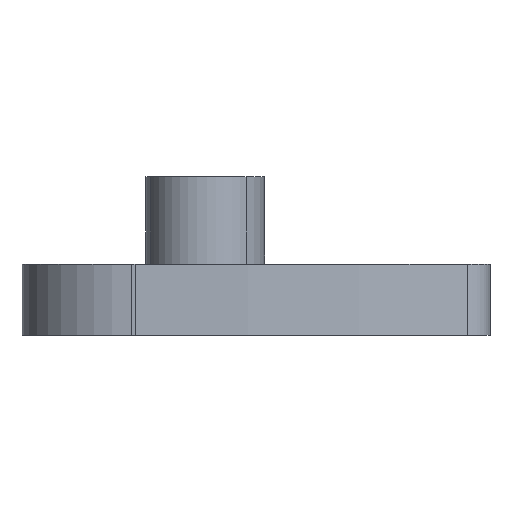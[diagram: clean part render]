
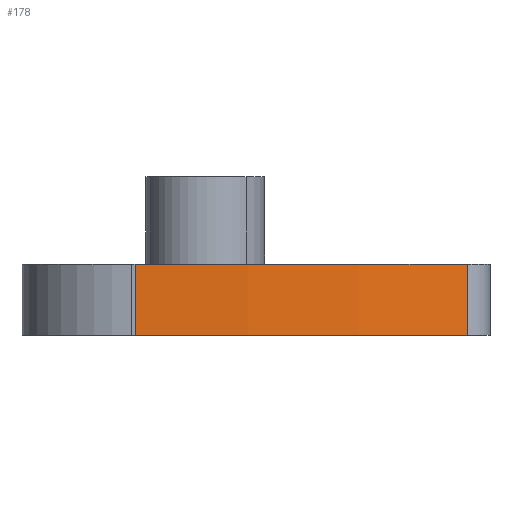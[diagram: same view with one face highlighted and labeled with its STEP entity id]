
A CAD part, left-side view. The second image highlights one B-rep face of the part: STEP entity #178.
In plain terms, the highlighted cylindrical face has radius 51.721 mm (diameter 103.442 mm), a partial arc.
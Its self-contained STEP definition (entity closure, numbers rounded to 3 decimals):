
#3 = AXIS2_PLACEMENT_3D ( 'NONE', #435, #183, #52 ) ;
#4 = CARTESIAN_POINT ( 'NONE',  ( -4.997, -12.663, 3.25 ) ) ;
#16 = DIRECTION ( 'NONE',  ( 0., 0., 1. ) ) ;
#52 = DIRECTION ( 'NONE',  ( 1., 0., 0. ) ) ;
#56 = VECTOR ( 'NONE', #476, 1000. ) ;
#168 = CIRCLE ( 'NONE', #233, 51.721 ) ;
#178 = ADVANCED_FACE ( 'NONE', ( #432 ), #405, .T. ) ;
#183 = DIRECTION ( 'NONE',  ( 0., 0., 1. ) ) ;
#191 = ORIENTED_EDGE ( 'NONE', *, *, #576, .T. ) ;
#193 = VERTEX_POINT ( 'NONE', #826 ) ;
#195 = DIRECTION ( 'NONE',  ( 0., 0., 1. ) ) ;
#225 = LINE ( 'NONE', #603, #56 ) ;
#229 = DIRECTION ( 'NONE',  ( 0., 0., 1. ) ) ;
#233 = AXIS2_PLACEMENT_3D ( 'NONE', #619, #229, #680 ) ;
#265 = LINE ( 'NONE', #471, #413 ) ;
#283 = ORIENTED_EDGE ( 'NONE', *, *, #602, .F. ) ;
#297 = CARTESIAN_POINT ( 'NONE',  ( -2.433, -27.845, 0. ) ) ;
#405 = CYLINDRICAL_SURFACE ( 'NONE', #3, 51.721 ) ;
#413 = VECTOR ( 'NONE', #16, 1000. ) ;
#432 = FACE_OUTER_BOUND ( 'NONE', #519, .T. ) ;
#435 = CARTESIAN_POINT ( 'NONE',  ( 46.715, -11.736, 0. ) ) ;
#437 = ORIENTED_EDGE ( 'NONE', *, *, #787, .F. ) ;
#464 = VERTEX_POINT ( 'NONE', #4 ) ;
#471 = CARTESIAN_POINT ( 'NONE',  ( -2.433, -27.845, 0. ) ) ;
#476 = DIRECTION ( 'NONE',  ( 0., 0., 1. ) ) ;
#519 = EDGE_LOOP ( 'NONE', ( #837, #191, #437, #283 ) ) ;
#576 = EDGE_CURVE ( 'NONE', #729, #825, #265, .T. ) ;
#584 = CARTESIAN_POINT ( 'NONE',  ( 46.715, -11.736, 3.25 ) ) ;
#588 = CARTESIAN_POINT ( 'NONE',  ( -2.433, -27.845, 3.25 ) ) ;
#602 = EDGE_CURVE ( 'NONE', #193, #464, #225, .T. ) ;
#603 = CARTESIAN_POINT ( 'NONE',  ( -4.997, -12.663, 0. ) ) ;
#619 = CARTESIAN_POINT ( 'NONE',  ( 46.715, -11.736, 0. ) ) ;
#647 = DIRECTION ( 'NONE',  ( 1., 0., 0. ) ) ;
#680 = DIRECTION ( 'NONE',  ( 1., 0., 0. ) ) ;
#689 = AXIS2_PLACEMENT_3D ( 'NONE', #584, #195, #647 ) ;
#723 = EDGE_CURVE ( 'NONE', #193, #729, #168, .T. ) ;
#729 = VERTEX_POINT ( 'NONE', #297 ) ;
#787 = EDGE_CURVE ( 'NONE', #464, #825, #790, .T. ) ;
#790 = CIRCLE ( 'NONE', #689, 51.721 ) ;
#825 = VERTEX_POINT ( 'NONE', #588 ) ;
#826 = CARTESIAN_POINT ( 'NONE',  ( -4.997, -12.663, 0. ) ) ;
#837 = ORIENTED_EDGE ( 'NONE', *, *, #723, .T. ) ;
